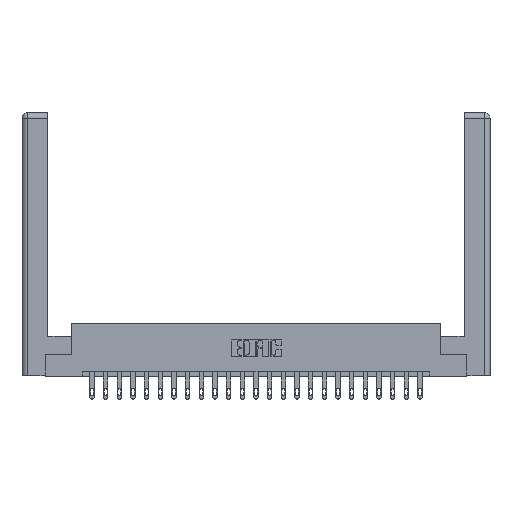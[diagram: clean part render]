
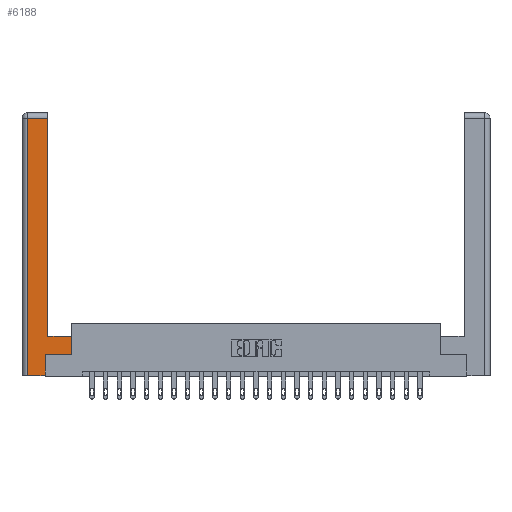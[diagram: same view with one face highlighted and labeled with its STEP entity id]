
A CAD part, top view. The second image highlights one B-rep face of the part: STEP entity #6188.
In plain terms, the highlighted planar face has unit normal (0, 0, 1).
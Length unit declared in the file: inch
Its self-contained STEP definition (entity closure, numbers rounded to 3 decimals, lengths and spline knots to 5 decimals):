
#100 = VERTEX_POINT ( 'NONE', #1913 ) ;
#264 = DIRECTION ( 'NONE',  ( -1., 0., 0. ) ) ;
#297 = VECTOR ( 'NONE', #23916, 39.37008 ) ;
#374 = EDGE_CURVE ( 'NONE', #1454, #13386, #14872, .T. ) ;
#557 = DIRECTION ( 'NONE',  ( 0., 1., 0. ) ) ;
#941 = CARTESIAN_POINT ( 'NONE',  ( 0.265, 0., 0. ) ) ;
#978 = LINE ( 'NONE', #21732, #4752 ) ;
#1454 = VERTEX_POINT ( 'NONE', #15300 ) ;
#1476 = DIRECTION ( 'NONE',  ( 0., 0., -1. ) ) ;
#1913 = CARTESIAN_POINT ( 'NONE',  ( 0.295, 2.94, 0. ) ) ;
#2732 = LINE ( 'NONE', #14842, #22857 ) ;
#3445 = DIRECTION ( 'NONE',  ( 1., 0., 0. ) ) ;
#3883 = ORIENTED_EDGE ( 'NONE', *, *, #14335, .T. ) ;
#4085 = VECTOR ( 'NONE', #264, 39.37008 ) ;
#4154 = DIRECTION ( 'NONE',  ( 0., 1., 0. ) ) ;
#4494 = EDGE_CURVE ( 'NONE', #13386, #18195, #8286, .T. ) ;
#4648 = EDGE_LOOP ( 'NONE', ( #16499, #14497, #13723, #20852, #9095, #3883, #18151, #12953 ) ) ;
#4752 = VECTOR ( 'NONE', #4959, 39.37008 ) ;
#4959 = DIRECTION ( 'NONE',  ( -1., 0., 0. ) ) ;
#5005 = CARTESIAN_POINT ( 'NONE',  ( 0.265, 0.245, 0. ) ) ;
#5143 = PLANE ( 'NONE',  #7000 ) ;
#5880 = LINE ( 'NONE', #22811, #9042 ) ;
#6188 = ADVANCED_FACE ( 'NONE', ( #15165 ), #5143, .F. ) ;
#6983 = EDGE_CURVE ( 'NONE', #22170, #12137, #13973, .T. ) ;
#7000 = AXIS2_PLACEMENT_3D ( 'NONE', #22168, #1476, #14909 ) ;
#8286 = LINE ( 'NONE', #941, #18446 ) ;
#8348 = DIRECTION ( 'NONE',  ( 0., -1., 0. ) ) ;
#8586 = EDGE_CURVE ( 'NONE', #18195, #21007, #22957, .T. ) ;
#9042 = VECTOR ( 'NONE', #4154, 39.37008 ) ;
#9095 = ORIENTED_EDGE ( 'NONE', *, *, #8586, .T. ) ;
#9407 = CARTESIAN_POINT ( 'NONE',  ( 0.0615, 0., 0. ) ) ;
#9955 = VECTOR ( 'NONE', #8348, 39.37008 ) ;
#10153 = DIRECTION ( 'NONE',  ( 1., 0., 0. ) ) ;
#11778 = EDGE_CURVE ( 'NONE', #12137, #13046, #21809, .T. ) ;
#12137 = VERTEX_POINT ( 'NONE', #19826 ) ;
#12512 = CARTESIAN_POINT ( 'NONE',  ( 0.295, 0.45, 0. ) ) ;
#12953 = ORIENTED_EDGE ( 'NONE', *, *, #11778, .T. ) ;
#13009 = CARTESIAN_POINT ( 'NONE',  ( 0.565, 0.245, 0. ) ) ;
#13046 = VERTEX_POINT ( 'NONE', #12512 ) ;
#13386 = VERTEX_POINT ( 'NONE', #9407 ) ;
#13723 = ORIENTED_EDGE ( 'NONE', *, *, #374, .T. ) ;
#13863 = CARTESIAN_POINT ( 'NONE',  ( 0.295, 0.45, 0. ) ) ;
#13973 = LINE ( 'NONE', #16213, #297 ) ;
#14166 = EDGE_CURVE ( 'NONE', #100, #1454, #978, .T. ) ;
#14335 = EDGE_CURVE ( 'NONE', #21007, #22170, #2732, .T. ) ;
#14497 = ORIENTED_EDGE ( 'NONE', *, *, #14166, .T. ) ;
#14842 = CARTESIAN_POINT ( 'NONE',  ( 0.565, 0.245, 0. ) ) ;
#14872 = LINE ( 'NONE', #19484, #9955 ) ;
#14909 = DIRECTION ( 'NONE',  ( -1., 0., 0. ) ) ;
#15165 = FACE_OUTER_BOUND ( 'NONE', #4648, .T. ) ;
#15300 = CARTESIAN_POINT ( 'NONE',  ( 0.0615, 2.94, 0. ) ) ;
#15533 = CARTESIAN_POINT ( 'NONE',  ( 0.265, 0., 0. ) ) ;
#16213 = CARTESIAN_POINT ( 'NONE',  ( 0.565, 0.45, 0. ) ) ;
#16499 = ORIENTED_EDGE ( 'NONE', *, *, #22961, .T. ) ;
#17382 = VECTOR ( 'NONE', #557, 39.37008 ) ;
#18151 = ORIENTED_EDGE ( 'NONE', *, *, #6983, .T. ) ;
#18195 = VERTEX_POINT ( 'NONE', #15533 ) ;
#18446 = VECTOR ( 'NONE', #10153, 39.37008 ) ;
#19484 = CARTESIAN_POINT ( 'NONE',  ( 0.0615, 0., 0. ) ) ;
#19826 = CARTESIAN_POINT ( 'NONE',  ( 0.565, 0.45, 0. ) ) ;
#20403 = CARTESIAN_POINT ( 'NONE',  ( 0.265, 0.245, 0. ) ) ;
#20852 = ORIENTED_EDGE ( 'NONE', *, *, #4494, .T. ) ;
#21007 = VERTEX_POINT ( 'NONE', #5005 ) ;
#21732 = CARTESIAN_POINT ( 'NONE',  ( 0.0615, 2.94, 0. ) ) ;
#21809 = LINE ( 'NONE', #13863, #4085 ) ;
#22168 = CARTESIAN_POINT ( 'NONE',  ( 0., 0., 0. ) ) ;
#22170 = VERTEX_POINT ( 'NONE', #13009 ) ;
#22811 = CARTESIAN_POINT ( 'NONE',  ( 0.295, 3., 0. ) ) ;
#22857 = VECTOR ( 'NONE', #3445, 39.37008 ) ;
#22957 = LINE ( 'NONE', #20403, #17382 ) ;
#22961 = EDGE_CURVE ( 'NONE', #13046, #100, #5880, .T. ) ;
#23916 = DIRECTION ( 'NONE',  ( 0., 1., 0. ) ) ;
